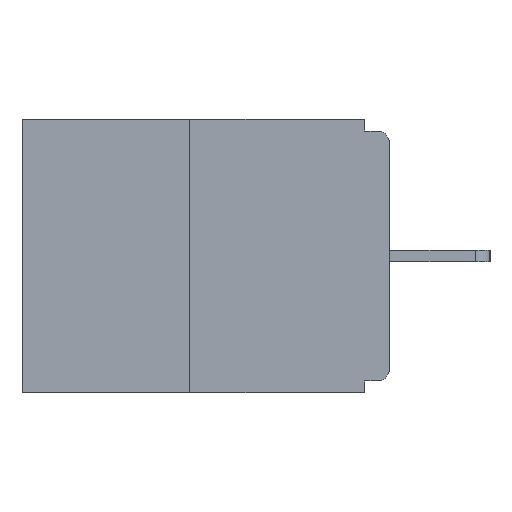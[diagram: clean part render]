
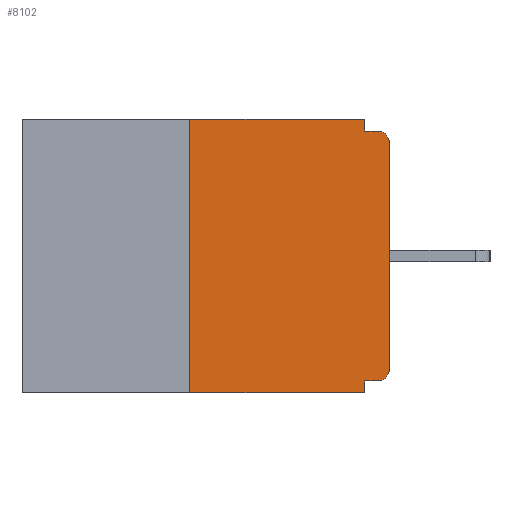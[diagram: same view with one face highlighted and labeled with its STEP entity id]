
A CAD part, left-side view. The second image highlights one B-rep face of the part: STEP entity #8102.
In plain terms, the highlighted planar face has unit normal (-1, 0, 0).
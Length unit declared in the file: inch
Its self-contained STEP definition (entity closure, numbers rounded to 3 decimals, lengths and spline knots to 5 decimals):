
#46 = DIRECTION ( 'NONE',  ( 0., 0., 1. ) ) ;
#51 = LINE ( 'NONE', #6646, #1351 ) ;
#115 = EDGE_CURVE ( 'NONE', #1842, #9353, #6704, .T. ) ;
#227 = CARTESIAN_POINT ( 'NONE',  ( 0., 0., -0.015 ) ) ;
#415 = DIRECTION ( 'NONE',  ( 0., -1., 0. ) ) ;
#646 = CARTESIAN_POINT ( 'NONE',  ( 0., 0., -0.328 ) ) ;
#786 = DIRECTION ( 'NONE',  ( 0., 1., 0. ) ) ;
#1219 = ORIENTED_EDGE ( 'NONE', *, *, #2064, .F. ) ;
#1333 = CARTESIAN_POINT ( 'NONE',  ( 0., 0.015, -0.03 ) ) ;
#1351 = VECTOR ( 'NONE', #2063, 39.37008 ) ;
#1455 = VERTEX_POINT ( 'NONE', #12141 ) ;
#1555 = EDGE_CURVE ( 'NONE', #3819, #6362, #11477, .T. ) ;
#1842 = VERTEX_POINT ( 'NONE', #2120 ) ;
#2008 = ORIENTED_EDGE ( 'NONE', *, *, #13797, .T. ) ;
#2063 = DIRECTION ( 'NONE',  ( 0., 0., -1. ) ) ;
#2064 = EDGE_CURVE ( 'NONE', #9353, #7246, #9538, .T. ) ;
#2120 = CARTESIAN_POINT ( 'NONE',  ( 0., 0.015, -0.328 ) ) ;
#2313 = CARTESIAN_POINT ( 'NONE',  ( 0., 0.015, -0.015 ) ) ;
#2681 = DIRECTION ( 'NONE',  ( 0., 0., -1. ) ) ;
#2969 = EDGE_CURVE ( 'NONE', #3021, #6622, #4747, .T. ) ;
#3021 = VERTEX_POINT ( 'NONE', #3546 ) ;
#3400 = ORIENTED_EDGE ( 'NONE', *, *, #7092, .F. ) ;
#3546 = CARTESIAN_POINT ( 'NONE',  ( 0., 0.25, -0.343 ) ) ;
#3614 = CARTESIAN_POINT ( 'NONE',  ( 0., 0., 0. ) ) ;
#3664 = ORIENTED_EDGE ( 'NONE', *, *, #9494, .T. ) ;
#3819 = VERTEX_POINT ( 'NONE', #10201 ) ;
#3882 = CARTESIAN_POINT ( 'NONE',  ( 0., 0., -0.03 ) ) ;
#3893 = VECTOR ( 'NONE', #46, 39.37008 ) ;
#4136 = CARTESIAN_POINT ( 'NONE',  ( 0., 0.031, -0.015 ) ) ;
#4469 = CARTESIAN_POINT ( 'NONE',  ( 0., 0.25, 0. ) ) ;
#4747 = LINE ( 'NONE', #14656, #14328 ) ;
#4820 = CARTESIAN_POINT ( 'NONE',  ( 0., 0.031, -0.343 ) ) ;
#4925 = DIRECTION ( 'NONE',  ( 1., 0., 0. ) ) ;
#5114 = CIRCLE ( 'NONE', #13370, 0.015 ) ;
#5320 = VECTOR ( 'NONE', #11613, 39.37008 ) ;
#5700 = DIRECTION ( 'NONE',  ( 0., -1., 0. ) ) ;
#6362 = VERTEX_POINT ( 'NONE', #3882 ) ;
#6420 = ORIENTED_EDGE ( 'NONE', *, *, #14634, .F. ) ;
#6622 = VERTEX_POINT ( 'NONE', #4469 ) ;
#6646 = CARTESIAN_POINT ( 'NONE',  ( 0., 0.031, 0. ) ) ;
#6704 = LINE ( 'NONE', #646, #11117 ) ;
#6728 = LINE ( 'NONE', #227, #10528 ) ;
#6869 = ORIENTED_EDGE ( 'NONE', *, *, #10725, .F. ) ;
#7092 = EDGE_CURVE ( 'NONE', #1455, #14438, #51, .T. ) ;
#7246 = VERTEX_POINT ( 'NONE', #4820 ) ;
#8051 = VERTEX_POINT ( 'NONE', #2313 ) ;
#8102 = ADVANCED_FACE ( 'NONE', ( #14080 ), #11726, .F. ) ;
#8615 = DIRECTION ( 'NONE',  ( 0., 0., -1. ) ) ;
#9266 = DIRECTION ( 'NONE',  ( 0., 0., 1. ) ) ;
#9353 = VERTEX_POINT ( 'NONE', #10709 ) ;
#9455 = DIRECTION ( 'NONE',  ( 0., 0., -1. ) ) ;
#9494 = EDGE_CURVE ( 'NONE', #1842, #3819, #11797, .T. ) ;
#9534 = ORIENTED_EDGE ( 'NONE', *, *, #2969, .F. ) ;
#9538 = LINE ( 'NONE', #12713, #5320 ) ;
#9583 = CARTESIAN_POINT ( 'NONE',  ( 0., 0.46, 0. ) ) ;
#9635 = CARTESIAN_POINT ( 'NONE',  ( 0., 0.46, -0.343 ) ) ;
#9930 = DIRECTION ( 'NONE',  ( 0., -1., 0. ) ) ;
#9955 = CARTESIAN_POINT ( 'NONE',  ( 0., 0.015, -0.313 ) ) ;
#10201 = CARTESIAN_POINT ( 'NONE',  ( 0., 0., -0.313 ) ) ;
#10225 = ORIENTED_EDGE ( 'NONE', *, *, #11479, .T. ) ;
#10426 = DIRECTION ( 'NONE',  ( -1., 0., 0. ) ) ;
#10528 = VECTOR ( 'NONE', #5700, 39.37008 ) ;
#10709 = CARTESIAN_POINT ( 'NONE',  ( 0., 0.031, -0.328 ) ) ;
#10725 = EDGE_CURVE ( 'NONE', #14438, #8051, #6728, .T. ) ;
#11117 = VECTOR ( 'NONE', #786, 39.37008 ) ;
#11411 = ORIENTED_EDGE ( 'NONE', *, *, #115, .F. ) ;
#11477 = LINE ( 'NONE', #3614, #3893 ) ;
#11479 = EDGE_CURVE ( 'NONE', #3021, #7246, #13025, .T. ) ;
#11613 = DIRECTION ( 'NONE',  ( 0., 0., -1. ) ) ;
#11726 = PLANE ( 'NONE',  #13646 ) ;
#11797 = CIRCLE ( 'NONE', #13208, 0.015 ) ;
#12141 = CARTESIAN_POINT ( 'NONE',  ( 0., 0.031, 0. ) ) ;
#12223 = DIRECTION ( 'NONE',  ( -1., 0., 0. ) ) ;
#12713 = CARTESIAN_POINT ( 'NONE',  ( 0., 0.031, -0.343 ) ) ;
#13025 = LINE ( 'NONE', #9635, #13550 ) ;
#13208 = AXIS2_PLACEMENT_3D ( 'NONE', #9955, #12223, #8615 ) ;
#13370 = AXIS2_PLACEMENT_3D ( 'NONE', #1333, #10426, #9455 ) ;
#13550 = VECTOR ( 'NONE', #9930, 39.37008 ) ;
#13646 = AXIS2_PLACEMENT_3D ( 'NONE', #9583, #4925, #2681 ) ;
#13690 = LINE ( 'NONE', #13758, #14553 ) ;
#13758 = CARTESIAN_POINT ( 'NONE',  ( 0., 0.46, 0. ) ) ;
#13777 = ORIENTED_EDGE ( 'NONE', *, *, #1555, .T. ) ;
#13797 = EDGE_CURVE ( 'NONE', #6362, #8051, #5114, .T. ) ;
#14038 = EDGE_LOOP ( 'NONE', ( #6420, #9534, #10225, #1219, #11411, #3664, #13777, #2008, #6869, #3400 ) ) ;
#14080 = FACE_OUTER_BOUND ( 'NONE', #14038, .T. ) ;
#14328 = VECTOR ( 'NONE', #9266, 39.37008 ) ;
#14438 = VERTEX_POINT ( 'NONE', #4136 ) ;
#14553 = VECTOR ( 'NONE', #415, 39.37008 ) ;
#14634 = EDGE_CURVE ( 'NONE', #6622, #1455, #13690, .T. ) ;
#14656 = CARTESIAN_POINT ( 'NONE',  ( 0., 0.25, 0. ) ) ;
